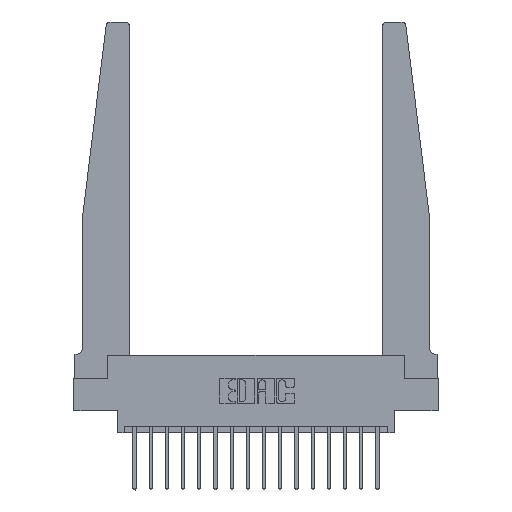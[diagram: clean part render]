
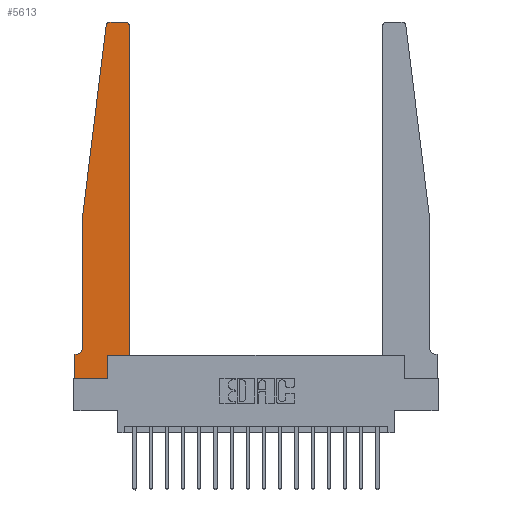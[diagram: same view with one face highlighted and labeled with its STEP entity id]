
A CAD part, top view. The second image highlights one B-rep face of the part: STEP entity #5613.
In plain terms, the highlighted planar face has unit normal (0, 0, 1).
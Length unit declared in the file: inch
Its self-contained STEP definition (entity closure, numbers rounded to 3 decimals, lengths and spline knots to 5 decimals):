
#34 = CARTESIAN_POINT ( 'NONE',  ( 0.27653, 2.72, 0.37 ) ) ;
#80 = LINE ( 'NONE', #18366, #7433 ) ;
#123 = LINE ( 'NONE', #7391, #15213 ) ;
#155 = DIRECTION ( 'NONE',  ( 0., 0., 1. ) ) ;
#257 = ORIENTED_EDGE ( 'NONE', *, *, #7300, .T. ) ;
#441 = CARTESIAN_POINT ( 'NONE',  ( 0., 0., 0.37 ) ) ;
#556 = PLANE ( 'NONE',  #11852 ) ;
#792 = AXIS2_PLACEMENT_3D ( 'NONE', #34, #10297, #1541 ) ;
#950 = CARTESIAN_POINT ( 'NONE',  ( 0., 0., 0.37 ) ) ;
#1001 = CARTESIAN_POINT ( 'NONE',  ( 0.065, 1.25, 0.37 ) ) ;
#1198 = EDGE_CURVE ( 'NONE', #18848, #1402, #11230, .T. ) ;
#1359 = AXIS2_PLACEMENT_3D ( 'NONE', #8933, #155, #10404 ) ;
#1402 = VERTEX_POINT ( 'NONE', #11385 ) ;
#1403 = CARTESIAN_POINT ( 'NONE',  ( 0.27653, 2.75, 0.37 ) ) ;
#1541 = DIRECTION ( 'NONE',  ( 1., 0., 0. ) ) ;
#1600 = VERTEX_POINT ( 'NONE', #7512 ) ;
#1974 = EDGE_CURVE ( 'NONE', #1402, #2491, #10099, .T. ) ;
#2087 = ORIENTED_EDGE ( 'NONE', *, *, #1974, .T. ) ;
#2176 = EDGE_CURVE ( 'NONE', #6014, #6601, #3498, .T. ) ;
#2316 = VECTOR ( 'NONE', #9784, 39.37008 ) ;
#2371 = DIRECTION ( 'NONE',  ( 0., 0., -1. ) ) ;
#2491 = VERTEX_POINT ( 'NONE', #5194 ) ;
#2508 = ORIENTED_EDGE ( 'NONE', *, *, #15911, .T. ) ;
#3498 = CIRCLE ( 'NONE', #792, 0.03 ) ;
#3529 = ORIENTED_EDGE ( 'NONE', *, *, #6101, .T. ) ;
#3703 = EDGE_CURVE ( 'NONE', #12161, #18848, #15056, .T. ) ;
#4074 = EDGE_CURVE ( 'NONE', #6601, #12160, #17731, .T. ) ;
#4606 = LINE ( 'NONE', #441, #8889 ) ;
#4813 = LINE ( 'NONE', #16491, #15928 ) ;
#4894 = ORIENTED_EDGE ( 'NONE', *, *, #13539, .T. ) ;
#5194 = CARTESIAN_POINT ( 'NONE',  ( 0., 0., 0.37 ) ) ;
#5613 = ADVANCED_FACE ( 'NONE', ( #12920 ), #556, .T. ) ;
#5682 = CARTESIAN_POINT ( 'NONE',  ( 0.395, 2.75, 0.37 ) ) ;
#6014 = VERTEX_POINT ( 'NONE', #1403 ) ;
#6083 = VECTOR ( 'NONE', #11611, 39.37008 ) ;
#6088 = CIRCLE ( 'NONE', #1359, 0.03 ) ;
#6101 = EDGE_CURVE ( 'NONE', #9526, #18242, #6088, .T. ) ;
#6310 = DIRECTION ( 'NONE',  ( 0., 1., 0. ) ) ;
#6461 = DIRECTION ( 'NONE',  ( 1., 0., 0. ) ) ;
#6510 = LINE ( 'NONE', #17454, #6083 ) ;
#6528 = ORIENTED_EDGE ( 'NONE', *, *, #2176, .T. ) ;
#6601 = VERTEX_POINT ( 'NONE', #11654 ) ;
#6627 = VERTEX_POINT ( 'NONE', #11833 ) ;
#7300 = EDGE_CURVE ( 'NONE', #12160, #12161, #11034, .T. ) ;
#7391 = CARTESIAN_POINT ( 'NONE',  ( 0.25, 2.75, 0.37 ) ) ;
#7433 = VECTOR ( 'NONE', #12607, 39.37008 ) ;
#7512 = CARTESIAN_POINT ( 'NONE',  ( 0.2605, 0.18, 0.37 ) ) ;
#7991 = CARTESIAN_POINT ( 'NONE',  ( 0.425, 0.18, 0.37 ) ) ;
#8355 = CARTESIAN_POINT ( 'NONE',  ( 0.425, 2.72, 0.37 ) ) ;
#8889 = VECTOR ( 'NONE', #12127, 39.37008 ) ;
#8933 = CARTESIAN_POINT ( 'NONE',  ( 0.395, 2.72, 0.37 ) ) ;
#9526 = VERTEX_POINT ( 'NONE', #8355 ) ;
#9628 = CARTESIAN_POINT ( 'NONE',  ( 0.065, 0.1875, 0.37 ) ) ;
#9784 = DIRECTION ( 'NONE',  ( 0., -1., 0. ) ) ;
#10026 = VECTOR ( 'NONE', #18450, 39.37008 ) ;
#10062 = CARTESIAN_POINT ( 'NONE',  ( 0.065, 0.2375, 0.37 ) ) ;
#10099 = LINE ( 'NONE', #950, #2316 ) ;
#10297 = DIRECTION ( 'NONE',  ( 0., 0., 1. ) ) ;
#10298 = CARTESIAN_POINT ( 'NONE',  ( 0.015, 0.1875, 0.37 ) ) ;
#10404 = DIRECTION ( 'NONE',  ( 1., 0., 0. ) ) ;
#10467 = ORIENTED_EDGE ( 'NONE', *, *, #11793, .T. ) ;
#10520 = EDGE_CURVE ( 'NONE', #2491, #6627, #4606, .T. ) ;
#11034 = LINE ( 'NONE', #12776, #18289 ) ;
#11105 = CARTESIAN_POINT ( 'NONE',  ( 0.015, 0.2375, 0.37 ) ) ;
#11230 = LINE ( 'NONE', #9628, #15133 ) ;
#11365 = DIRECTION ( 'NONE',  ( 0., -1., 0. ) ) ;
#11385 = CARTESIAN_POINT ( 'NONE',  ( 0., 0.1875, 0.37 ) ) ;
#11611 = DIRECTION ( 'NONE',  ( 1., 0., 0. ) ) ;
#11654 = CARTESIAN_POINT ( 'NONE',  ( 0.24675, 2.72367, 0.37 ) ) ;
#11767 = DIRECTION ( 'NONE',  ( -1., 0., 0. ) ) ;
#11793 = EDGE_CURVE ( 'NONE', #13433, #9526, #4813, .T. ) ;
#11833 = CARTESIAN_POINT ( 'NONE',  ( 0.2605, 0., 0.37 ) ) ;
#11852 = AXIS2_PLACEMENT_3D ( 'NONE', #12239, #15187, #6461 ) ;
#12127 = DIRECTION ( 'NONE',  ( 1., 0., 0. ) ) ;
#12160 = VERTEX_POINT ( 'NONE', #18722 ) ;
#12161 = VERTEX_POINT ( 'NONE', #10062 ) ;
#12239 = CARTESIAN_POINT ( 'NONE',  ( 0., 0.1875, 0.37 ) ) ;
#12507 = ORIENTED_EDGE ( 'NONE', *, *, #3703, .T. ) ;
#12574 = DIRECTION ( 'NONE',  ( -1., 0., 0. ) ) ;
#12607 = DIRECTION ( 'NONE',  ( 0., 1., 0. ) ) ;
#12776 = CARTESIAN_POINT ( 'NONE',  ( 0.065, 1.25, 0.37 ) ) ;
#12920 = FACE_OUTER_BOUND ( 'NONE', #15711, .T. ) ;
#13070 = AXIS2_PLACEMENT_3D ( 'NONE', #11105, #2371, #12574 ) ;
#13433 = VERTEX_POINT ( 'NONE', #7991 ) ;
#13539 = EDGE_CURVE ( 'NONE', #6627, #1600, #80, .T. ) ;
#14109 = ORIENTED_EDGE ( 'NONE', *, *, #16967, .T. ) ;
#15056 = CIRCLE ( 'NONE', #13070, 0.05 ) ;
#15078 = ORIENTED_EDGE ( 'NONE', *, *, #1198, .T. ) ;
#15133 = VECTOR ( 'NONE', #18282, 39.37008 ) ;
#15187 = DIRECTION ( 'NONE',  ( 0., 0., 1. ) ) ;
#15213 = VECTOR ( 'NONE', #11767, 39.37008 ) ;
#15294 = ORIENTED_EDGE ( 'NONE', *, *, #10520, .T. ) ;
#15711 = EDGE_LOOP ( 'NONE', ( #2508, #6528, #18618, #257, #12507, #15078, #2087, #15294, #4894, #14109, #10467, #3529 ) ) ;
#15911 = EDGE_CURVE ( 'NONE', #18242, #6014, #123, .T. ) ;
#15928 = VECTOR ( 'NONE', #6310, 39.37008 ) ;
#16491 = CARTESIAN_POINT ( 'NONE',  ( 0.425, 0.18, 0.37 ) ) ;
#16967 = EDGE_CURVE ( 'NONE', #1600, #13433, #6510, .T. ) ;
#17454 = CARTESIAN_POINT ( 'NONE',  ( 0.425, 0.18, 0.37 ) ) ;
#17731 = LINE ( 'NONE', #1001, #10026 ) ;
#18242 = VERTEX_POINT ( 'NONE', #5682 ) ;
#18282 = DIRECTION ( 'NONE',  ( -1., 0., 0. ) ) ;
#18289 = VECTOR ( 'NONE', #11365, 39.37008 ) ;
#18366 = CARTESIAN_POINT ( 'NONE',  ( 0.2605, 0.18, 0.37 ) ) ;
#18450 = DIRECTION ( 'NONE',  ( -0.122, -0.992, 0. ) ) ;
#18618 = ORIENTED_EDGE ( 'NONE', *, *, #4074, .T. ) ;
#18722 = CARTESIAN_POINT ( 'NONE',  ( 0.065, 1.25, 0.37 ) ) ;
#18848 = VERTEX_POINT ( 'NONE', #10298 ) ;
